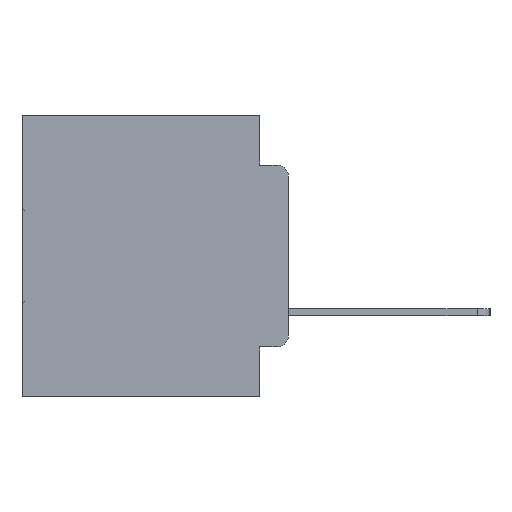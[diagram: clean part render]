
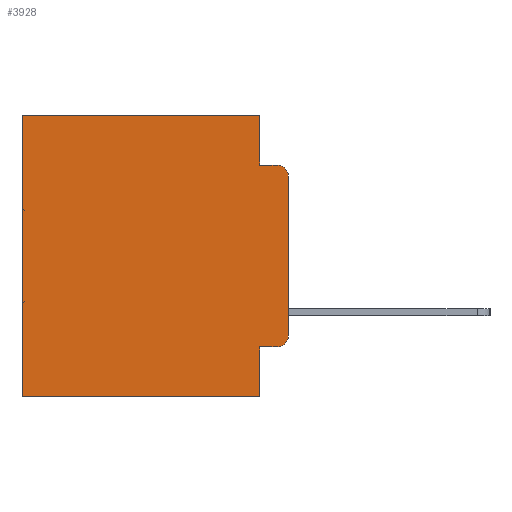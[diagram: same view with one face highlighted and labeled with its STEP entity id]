
A CAD part, left-side view. The second image highlights one B-rep face of the part: STEP entity #3928.
In plain terms, the highlighted planar face has unit normal (-1, 0, 0).
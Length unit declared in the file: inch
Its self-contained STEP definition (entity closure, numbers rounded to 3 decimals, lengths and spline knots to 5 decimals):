
#34 = VECTOR ( 'NONE', #22374, 39.37008 ) ;
#523 = EDGE_CURVE ( 'NONE', #12099, #17858, #1619, .T. ) ;
#1619 = LINE ( 'NONE', #5872, #34 ) ;
#1748 = DIRECTION ( 'NONE',  ( 0., -1., 0. ) ) ;
#1858 = VERTEX_POINT ( 'NONE', #23013 ) ;
#2143 = EDGE_CURVE ( 'NONE', #5765, #29823, #24677, .T. ) ;
#2500 = DIRECTION ( 'NONE',  ( 0., 0., -1. ) ) ;
#2561 = PLANE ( 'NONE',  #15482 ) ;
#2717 = ORIENTED_EDGE ( 'NONE', *, *, #26184, .T. ) ;
#3057 = EDGE_CURVE ( 'NONE', #5765, #21213, #25369, .T. ) ;
#3187 = DIRECTION ( 'NONE',  ( 0., 0., -1. ) ) ;
#3928 = ADVANCED_FACE ( 'NONE', ( #10794 ), #2561, .F. ) ;
#4042 = DIRECTION ( 'NONE',  ( 0., 0., -1. ) ) ;
#4190 = CARTESIAN_POINT ( 'NONE',  ( 0.298, 0., 0. ) ) ;
#4245 = ORIENTED_EDGE ( 'NONE', *, *, #28233, .T. ) ;
#4879 = VECTOR ( 'NONE', #22667, 39.37008 ) ;
#4883 = DIRECTION ( 'NONE',  ( 0., 0., -1. ) ) ;
#5407 = ORIENTED_EDGE ( 'NONE', *, *, #29590, .T. ) ;
#5765 = VERTEX_POINT ( 'NONE', #19808 ) ;
#5797 = ORIENTED_EDGE ( 'NONE', *, *, #3057, .F. ) ;
#5872 = CARTESIAN_POINT ( 'NONE',  ( 0.298, 0., 0. ) ) ;
#6390 = CARTESIAN_POINT ( 'NONE',  ( 0.298, 0.02, -0.4115 ) ) ;
#6555 = CARTESIAN_POINT ( 'NONE',  ( 0.298, 0., 0. ) ) ;
#7054 = VERTEX_POINT ( 'NONE', #27140 ) ;
#7256 = DIRECTION ( 'NONE',  ( 1., 0., 0. ) ) ;
#7353 = EDGE_CURVE ( 'NONE', #1858, #16511, #8249, .T. ) ;
#7414 = CARTESIAN_POINT ( 'NONE',  ( 0.298, 0.473, -0.5 ) ) ;
#7454 = VECTOR ( 'NONE', #18527, 39.37008 ) ;
#7736 = DIRECTION ( 'NONE',  ( -1., 0., 0. ) ) ;
#8249 = LINE ( 'NONE', #11038, #7454 ) ;
#9459 = CARTESIAN_POINT ( 'NONE',  ( 0.298, 0.051, 0. ) ) ;
#10794 = FACE_OUTER_BOUND ( 'NONE', #31185, .T. ) ;
#11038 = CARTESIAN_POINT ( 'NONE',  ( 0.298, 0., -0.5 ) ) ;
#11229 = CARTESIAN_POINT ( 'NONE',  ( 0.298, 0.473, 0. ) ) ;
#11762 = CARTESIAN_POINT ( 'NONE',  ( 0.298, 0.051, 0. ) ) ;
#12099 = VERTEX_POINT ( 'NONE', #11762 ) ;
#14018 = ORIENTED_EDGE ( 'NONE', *, *, #27473, .F. ) ;
#14543 = CARTESIAN_POINT ( 'NONE',  ( 0.298, 0.051, -0.0885 ) ) ;
#15025 = LINE ( 'NONE', #9459, #27138 ) ;
#15482 = AXIS2_PLACEMENT_3D ( 'NONE', #6555, #7256, #3187 ) ;
#15887 = LINE ( 'NONE', #31104, #27968 ) ;
#16373 = ORIENTED_EDGE ( 'NONE', *, *, #523, .T. ) ;
#16505 = EDGE_CURVE ( 'NONE', #12099, #29959, #15025, .T. ) ;
#16511 = VERTEX_POINT ( 'NONE', #7414 ) ;
#17496 = VECTOR ( 'NONE', #4883, 39.37008 ) ;
#17858 = VERTEX_POINT ( 'NONE', #11229 ) ;
#18102 = CARTESIAN_POINT ( 'NONE',  ( 0.298, 0.051, -0.0885 ) ) ;
#18527 = DIRECTION ( 'NONE',  ( 0., 1., 0. ) ) ;
#18604 = VECTOR ( 'NONE', #4042, 39.37008 ) ;
#18934 = LINE ( 'NONE', #29921, #4879 ) ;
#19646 = DIRECTION ( 'NONE',  ( -1., 0., 0. ) ) ;
#19673 = CARTESIAN_POINT ( 'NONE',  ( 0.298, 0.02, -0.1085 ) ) ;
#19713 = VERTEX_POINT ( 'NONE', #6390 ) ;
#19808 = CARTESIAN_POINT ( 'NONE',  ( 0.298, 0., -0.1085 ) ) ;
#20180 = ORIENTED_EDGE ( 'NONE', *, *, #21387, .F. ) ;
#20780 = DIRECTION ( 'NONE',  ( 0., 0., -1. ) ) ;
#21213 = VERTEX_POINT ( 'NONE', #24453 ) ;
#21294 = CARTESIAN_POINT ( 'NONE',  ( 0.298, 0.473, 0. ) ) ;
#21387 = EDGE_CURVE ( 'NONE', #7054, #1858, #18934, .T. ) ;
#22303 = CARTESIAN_POINT ( 'NONE',  ( 0.298, 0.02, -0.0885 ) ) ;
#22374 = DIRECTION ( 'NONE',  ( 0., 1., 0. ) ) ;
#22491 = CARTESIAN_POINT ( 'NONE',  ( 0.298, 0.02, -0.3915 ) ) ;
#22667 = DIRECTION ( 'NONE',  ( 0., 0., -1. ) ) ;
#23013 = CARTESIAN_POINT ( 'NONE',  ( 0.298, 0.051, -0.5 ) ) ;
#23747 = LINE ( 'NONE', #14543, #29392 ) ;
#23895 = AXIS2_PLACEMENT_3D ( 'NONE', #22491, #7736, #24885 ) ;
#24231 = LINE ( 'NONE', #21294, #18604 ) ;
#24453 = CARTESIAN_POINT ( 'NONE',  ( 0.298, 0., -0.3915 ) ) ;
#24677 = CIRCLE ( 'NONE', #25589, 0.02 ) ;
#24885 = DIRECTION ( 'NONE',  ( 0., 0., -1. ) ) ;
#25369 = LINE ( 'NONE', #4190, #17496 ) ;
#25589 = AXIS2_PLACEMENT_3D ( 'NONE', #19673, #19646, #20780 ) ;
#26184 = EDGE_CURVE ( 'NONE', #7054, #19713, #15887, .T. ) ;
#26567 = ORIENTED_EDGE ( 'NONE', *, *, #7353, .F. ) ;
#26926 = ORIENTED_EDGE ( 'NONE', *, *, #2143, .T. ) ;
#27138 = VECTOR ( 'NONE', #2500, 39.37008 ) ;
#27140 = CARTESIAN_POINT ( 'NONE',  ( 0.298, 0.051, -0.4115 ) ) ;
#27473 = EDGE_CURVE ( 'NONE', #29959, #29823, #23747, .T. ) ;
#27968 = VECTOR ( 'NONE', #1748, 39.37008 ) ;
#28233 = EDGE_CURVE ( 'NONE', #19713, #21213, #31568, .T. ) ;
#29152 = DIRECTION ( 'NONE',  ( 0., -1., 0. ) ) ;
#29197 = ORIENTED_EDGE ( 'NONE', *, *, #16505, .F. ) ;
#29392 = VECTOR ( 'NONE', #29152, 39.37008 ) ;
#29590 = EDGE_CURVE ( 'NONE', #17858, #16511, #24231, .T. ) ;
#29823 = VERTEX_POINT ( 'NONE', #22303 ) ;
#29921 = CARTESIAN_POINT ( 'NONE',  ( 0.298, 0.051, 0. ) ) ;
#29959 = VERTEX_POINT ( 'NONE', #18102 ) ;
#31104 = CARTESIAN_POINT ( 'NONE',  ( 0.298, 0.051, -0.4115 ) ) ;
#31185 = EDGE_LOOP ( 'NONE', ( #5797, #26926, #14018, #29197, #16373, #5407, #26567, #20180, #2717, #4245 ) ) ;
#31568 = CIRCLE ( 'NONE', #23895, 0.02 ) ;
